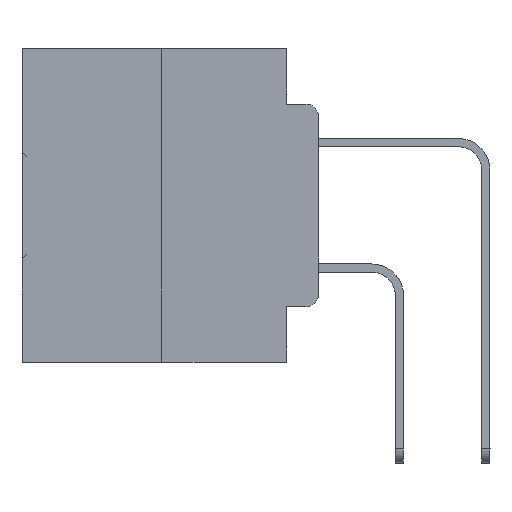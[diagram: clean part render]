
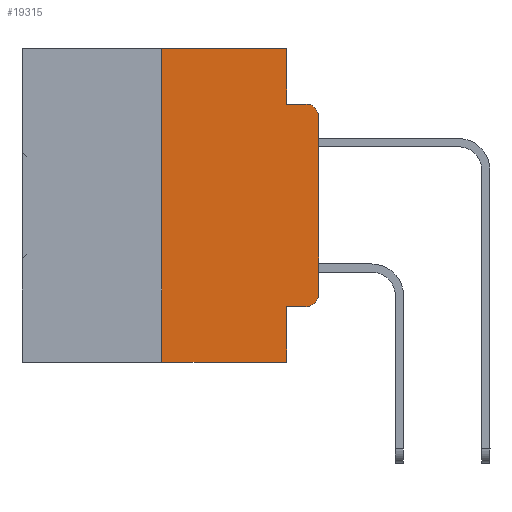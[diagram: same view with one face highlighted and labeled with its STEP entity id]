
A CAD part, left-side view. The second image highlights one B-rep face of the part: STEP entity #19315.
In plain terms, the highlighted planar face has unit normal (-1, 0, 0).
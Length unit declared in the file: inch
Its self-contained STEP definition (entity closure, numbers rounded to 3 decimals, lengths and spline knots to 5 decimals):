
#550 = AXIS2_PLACEMENT_3D ( 'NONE', #21071, #29504, #17797 ) ;
#796 = CARTESIAN_POINT ( 'NONE',  ( 0., 0.473, -0.5 ) ) ;
#1351 = VERTEX_POINT ( 'NONE', #6627 ) ;
#1737 = DIRECTION ( 'NONE',  ( 1., 0., 0. ) ) ;
#2296 = DIRECTION ( 'NONE',  ( 0., 0., -1. ) ) ;
#2803 = EDGE_CURVE ( 'NONE', #14525, #6550, #31637, .T. ) ;
#2829 = LINE ( 'NONE', #14031, #25072 ) ;
#4211 = CARTESIAN_POINT ( 'NONE',  ( 0., 0.051, -0.5 ) ) ;
#4383 = VECTOR ( 'NONE', #25456, 39.37008 ) ;
#6188 = LINE ( 'NONE', #14991, #6893 ) ;
#6337 = AXIS2_PLACEMENT_3D ( 'NONE', #26866, #1737, #32156 ) ;
#6550 = VERTEX_POINT ( 'NONE', #29169 ) ;
#6627 = CARTESIAN_POINT ( 'NONE',  ( 0., 0.02, -0.4115 ) ) ;
#6745 = VECTOR ( 'NONE', #32182, 39.37008 ) ;
#6893 = VECTOR ( 'NONE', #17935, 39.37008 ) ;
#7620 = CARTESIAN_POINT ( 'NONE',  ( 0., 0.051, 0. ) ) ;
#7718 = DIRECTION ( 'NONE',  ( -1., 0., 0. ) ) ;
#7891 = VERTEX_POINT ( 'NONE', #34735 ) ;
#8034 = EDGE_CURVE ( 'NONE', #24860, #14525, #2829, .T. ) ;
#8037 = LINE ( 'NONE', #19229, #24992 ) ;
#9279 = EDGE_CURVE ( 'NONE', #14524, #1351, #20841, .T. ) ;
#9571 = ORIENTED_EDGE ( 'NONE', *, *, #8034, .T. ) ;
#9818 = PLANE ( 'NONE',  #6337 ) ;
#9841 = CARTESIAN_POINT ( 'NONE',  ( 0., 0.25, -0.5 ) ) ;
#10284 = EDGE_CURVE ( 'NONE', #7891, #6550, #35911, .T. ) ;
#10536 = EDGE_CURVE ( 'NONE', #1351, #24860, #15766, .T. ) ;
#10805 = VECTOR ( 'NONE', #20396, 39.37008 ) ;
#10824 = DIRECTION ( 'NONE',  ( 0., -1., 0. ) ) ;
#11344 = ORIENTED_EDGE ( 'NONE', *, *, #2803, .T. ) ;
#11378 = ORIENTED_EDGE ( 'NONE', *, *, #18864, .F. ) ;
#13053 = ORIENTED_EDGE ( 'NONE', *, *, #29699, .F. ) ;
#13446 = ORIENTED_EDGE ( 'NONE', *, *, #10536, .T. ) ;
#13560 = CARTESIAN_POINT ( 'NONE',  ( 0., 0., -0.3915 ) ) ;
#13953 = DIRECTION ( 'NONE',  ( 0., 0., -1. ) ) ;
#14031 = CARTESIAN_POINT ( 'NONE',  ( 0., 0., 0. ) ) ;
#14102 = VERTEX_POINT ( 'NONE', #4211 ) ;
#14524 = VERTEX_POINT ( 'NONE', #21586 ) ;
#14525 = VERTEX_POINT ( 'NONE', #23794 ) ;
#14991 = CARTESIAN_POINT ( 'NONE',  ( 0., 0.473, 0. ) ) ;
#15033 = ORIENTED_EDGE ( 'NONE', *, *, #9279, .T. ) ;
#15766 = CIRCLE ( 'NONE', #550, 0.02 ) ;
#15873 = LINE ( 'NONE', #7620, #28870 ) ;
#16953 = CARTESIAN_POINT ( 'NONE',  ( 0., 0.051, 0. ) ) ;
#17797 = DIRECTION ( 'NONE',  ( 0., 0., -1. ) ) ;
#17935 = DIRECTION ( 'NONE',  ( 0., -1., 0. ) ) ;
#18864 = EDGE_CURVE ( 'NONE', #24937, #22106, #6188, .T. ) ;
#18922 = EDGE_LOOP ( 'NONE', ( #9571, #11344, #35011, #22393, #11378, #32130, #29884, #13053, #15033, #13446 ) ) ;
#19229 = CARTESIAN_POINT ( 'NONE',  ( 0., 0.051, 0. ) ) ;
#19315 = ADVANCED_FACE ( 'NONE', ( #26686 ), #9818, .F. ) ;
#19952 = LINE ( 'NONE', #30757, #4383 ) ;
#20396 = DIRECTION ( 'NONE',  ( 0., -1., 0. ) ) ;
#20841 = LINE ( 'NONE', #32002, #6745 ) ;
#21071 = CARTESIAN_POINT ( 'NONE',  ( 0., 0.02, -0.3915 ) ) ;
#21547 = DIRECTION ( 'NONE',  ( 0., 0., 1. ) ) ;
#21586 = CARTESIAN_POINT ( 'NONE',  ( 0., 0.051, -0.4115 ) ) ;
#22106 = VERTEX_POINT ( 'NONE', #16953 ) ;
#22393 = ORIENTED_EDGE ( 'NONE', *, *, #32315, .F. ) ;
#23794 = CARTESIAN_POINT ( 'NONE',  ( 0., 0., -0.1085 ) ) ;
#24551 = CARTESIAN_POINT ( 'NONE',  ( 0., 0.25, 0. ) ) ;
#24860 = VERTEX_POINT ( 'NONE', #13560 ) ;
#24937 = VERTEX_POINT ( 'NONE', #24551 ) ;
#24992 = VECTOR ( 'NONE', #34386, 39.37008 ) ;
#25072 = VECTOR ( 'NONE', #21547, 39.37008 ) ;
#25102 = EDGE_CURVE ( 'NONE', #32234, #24937, #19952, .T. ) ;
#25456 = DIRECTION ( 'NONE',  ( 0., 0., 1. ) ) ;
#25899 = LINE ( 'NONE', #796, #10805 ) ;
#26686 = FACE_OUTER_BOUND ( 'NONE', #18922, .T. ) ;
#26866 = CARTESIAN_POINT ( 'NONE',  ( 0., 0.473, 0. ) ) ;
#27559 = EDGE_CURVE ( 'NONE', #32234, #14102, #25899, .T. ) ;
#28870 = VECTOR ( 'NONE', #2296, 39.37008 ) ;
#29169 = CARTESIAN_POINT ( 'NONE',  ( 0., 0.02, -0.0885 ) ) ;
#29504 = DIRECTION ( 'NONE',  ( -1., 0., 0. ) ) ;
#29699 = EDGE_CURVE ( 'NONE', #14524, #14102, #8037, .T. ) ;
#29884 = ORIENTED_EDGE ( 'NONE', *, *, #27559, .T. ) ;
#30426 = CARTESIAN_POINT ( 'NONE',  ( 0., 0.051, -0.0885 ) ) ;
#30757 = CARTESIAN_POINT ( 'NONE',  ( 0., 0.25, 0. ) ) ;
#31063 = AXIS2_PLACEMENT_3D ( 'NONE', #36086, #7718, #13953 ) ;
#31637 = CIRCLE ( 'NONE', #31063, 0.02 ) ;
#32002 = CARTESIAN_POINT ( 'NONE',  ( 0., 0.051, -0.4115 ) ) ;
#32130 = ORIENTED_EDGE ( 'NONE', *, *, #25102, .F. ) ;
#32156 = DIRECTION ( 'NONE',  ( 0., 0., -1. ) ) ;
#32182 = DIRECTION ( 'NONE',  ( 0., -1., 0. ) ) ;
#32234 = VERTEX_POINT ( 'NONE', #9841 ) ;
#32315 = EDGE_CURVE ( 'NONE', #22106, #7891, #15873, .T. ) ;
#34386 = DIRECTION ( 'NONE',  ( 0., 0., -1. ) ) ;
#34735 = CARTESIAN_POINT ( 'NONE',  ( 0., 0.051, -0.0885 ) ) ;
#34929 = VECTOR ( 'NONE', #10824, 39.37008 ) ;
#35011 = ORIENTED_EDGE ( 'NONE', *, *, #10284, .F. ) ;
#35911 = LINE ( 'NONE', #30426, #34929 ) ;
#36086 = CARTESIAN_POINT ( 'NONE',  ( 0., 0.02, -0.1085 ) ) ;
